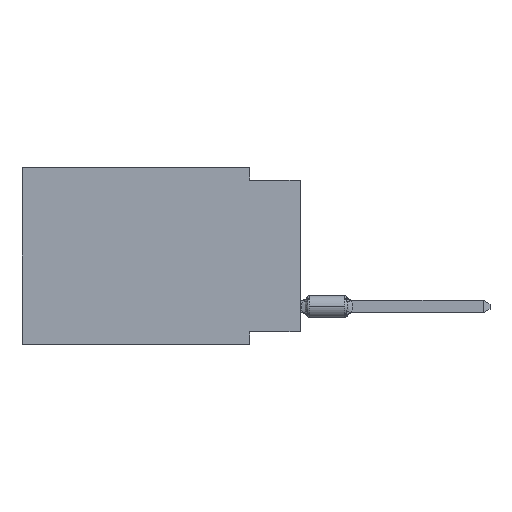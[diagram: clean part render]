
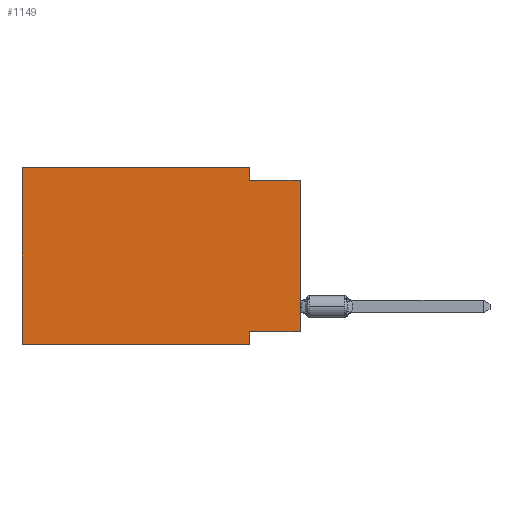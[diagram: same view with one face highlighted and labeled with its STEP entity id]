
A CAD part, left-side view. The second image highlights one B-rep face of the part: STEP entity #1149.
In plain terms, the highlighted planar face has unit normal (-1, 0, 0).
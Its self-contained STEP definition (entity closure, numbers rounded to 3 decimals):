
#193 = CARTESIAN_POINT ( 'NONE',  ( 0., 13.97, 0. ) ) ;
#929 = CARTESIAN_POINT ( 'NONE',  ( 0., 2.54, -8.89 ) ) ;
#1138 = CARTESIAN_POINT ( 'NONE',  ( 0., 13.97, 0. ) ) ;
#1149 = ADVANCED_FACE ( 'NONE', ( #1326 ), #18339, .F. ) ;
#1326 = FACE_OUTER_BOUND ( 'NONE', #17792, .T. ) ;
#1440 = ORIENTED_EDGE ( 'NONE', *, *, #24426, .F. ) ;
#1640 = DIRECTION ( 'NONE',  ( 0., 1., 0. ) ) ;
#1644 = ORIENTED_EDGE ( 'NONE', *, *, #5877, .F. ) ;
#1677 = VERTEX_POINT ( 'NONE', #9015 ) ;
#1721 = VECTOR ( 'NONE', #23499, 1000. ) ;
#2158 = VERTEX_POINT ( 'NONE', #929 ) ;
#2581 = CARTESIAN_POINT ( 'NONE',  ( 0., 0., -8.255 ) ) ;
#2941 = ORIENTED_EDGE ( 'NONE', *, *, #13775, .F. ) ;
#3769 = DIRECTION ( 'NONE',  ( 0., 0., 1. ) ) ;
#4730 = LINE ( 'NONE', #8954, #1721 ) ;
#5130 = VECTOR ( 'NONE', #18849, 1000. ) ;
#5492 = LINE ( 'NONE', #11740, #8200 ) ;
#5517 = DIRECTION ( 'NONE',  ( 0., -1., 0. ) ) ;
#5852 = EDGE_CURVE ( 'NONE', #6521, #20595, #18789, .T. ) ;
#5877 = EDGE_CURVE ( 'NONE', #26163, #13690, #10086, .T. ) ;
#6096 = CARTESIAN_POINT ( 'NONE',  ( 0., 0., 0. ) ) ;
#6145 = CARTESIAN_POINT ( 'NONE',  ( 0., 2.54, 0. ) ) ;
#6521 = VERTEX_POINT ( 'NONE', #19542 ) ;
#6709 = CARTESIAN_POINT ( 'NONE',  ( 0., 2.54, -0.635 ) ) ;
#7259 = DIRECTION ( 'NONE',  ( 0., -1., 0. ) ) ;
#8200 = VECTOR ( 'NONE', #12275, 1000. ) ;
#8643 = VERTEX_POINT ( 'NONE', #20209 ) ;
#8954 = CARTESIAN_POINT ( 'NONE',  ( 0., 0., -0.635 ) ) ;
#9015 = CARTESIAN_POINT ( 'NONE',  ( 0., 0., -0.635 ) ) ;
#9643 = DIRECTION ( 'NONE',  ( 0., 0., -1. ) ) ;
#9997 = EDGE_CURVE ( 'NONE', #8643, #16742, #10549, .T. ) ;
#10086 = LINE ( 'NONE', #12397, #16259 ) ;
#10549 = LINE ( 'NONE', #193, #5130 ) ;
#11740 = CARTESIAN_POINT ( 'NONE',  ( 0., 2.54, -8.89 ) ) ;
#11957 = LINE ( 'NONE', #6096, #15734 ) ;
#12275 = DIRECTION ( 'NONE',  ( 0., 0., -1. ) ) ;
#12353 = CARTESIAN_POINT ( 'NONE',  ( 0., 13.97, 0. ) ) ;
#12365 = VECTOR ( 'NONE', #26683, 1000. ) ;
#12397 = CARTESIAN_POINT ( 'NONE',  ( 0., 0., -8.255 ) ) ;
#12660 = AXIS2_PLACEMENT_3D ( 'NONE', #12353, #26641, #9643 ) ;
#12902 = ORIENTED_EDGE ( 'NONE', *, *, #9997, .F. ) ;
#13103 = EDGE_CURVE ( 'NONE', #16742, #6521, #19792, .T. ) ;
#13654 = CARTESIAN_POINT ( 'NONE',  ( 0., 13.97, -8.89 ) ) ;
#13690 = VERTEX_POINT ( 'NONE', #25284 ) ;
#13775 = EDGE_CURVE ( 'NONE', #20595, #1677, #4730, .T. ) ;
#15511 = ORIENTED_EDGE ( 'NONE', *, *, #13103, .F. ) ;
#15734 = VECTOR ( 'NONE', #3769, 1000. ) ;
#16259 = VECTOR ( 'NONE', #1640, 1000. ) ;
#16643 = ORIENTED_EDGE ( 'NONE', *, *, #17890, .T. ) ;
#16742 = VERTEX_POINT ( 'NONE', #22946 ) ;
#16917 = VECTOR ( 'NONE', #5517, 1000. ) ;
#17792 = EDGE_LOOP ( 'NONE', ( #16643, #2941, #26818, #15511, #12902, #22213, #1440, #1644 ) ) ;
#17890 = EDGE_CURVE ( 'NONE', #26163, #1677, #11957, .T. ) ;
#18339 = PLANE ( 'NONE',  #12660 ) ;
#18789 = LINE ( 'NONE', #6145, #12365 ) ;
#18849 = DIRECTION ( 'NONE',  ( 0., 0., 1. ) ) ;
#19542 = CARTESIAN_POINT ( 'NONE',  ( 0., 2.54, 0. ) ) ;
#19792 = LINE ( 'NONE', #1138, #16917 ) ;
#20209 = CARTESIAN_POINT ( 'NONE',  ( 0., 13.97, -8.89 ) ) ;
#20363 = VECTOR ( 'NONE', #7259, 1000. ) ;
#20595 = VERTEX_POINT ( 'NONE', #6709 ) ;
#22213 = ORIENTED_EDGE ( 'NONE', *, *, #24335, .T. ) ;
#22946 = CARTESIAN_POINT ( 'NONE',  ( 0., 13.97, 0. ) ) ;
#23499 = DIRECTION ( 'NONE',  ( 0., -1., 0. ) ) ;
#24335 = EDGE_CURVE ( 'NONE', #8643, #2158, #25768, .T. ) ;
#24426 = EDGE_CURVE ( 'NONE', #13690, #2158, #5492, .T. ) ;
#25284 = CARTESIAN_POINT ( 'NONE',  ( 0., 2.54, -8.255 ) ) ;
#25768 = LINE ( 'NONE', #13654, #20363 ) ;
#26163 = VERTEX_POINT ( 'NONE', #2581 ) ;
#26641 = DIRECTION ( 'NONE',  ( 1., 0., 0. ) ) ;
#26683 = DIRECTION ( 'NONE',  ( 0., 0., -1. ) ) ;
#26818 = ORIENTED_EDGE ( 'NONE', *, *, #5852, .F. ) ;
